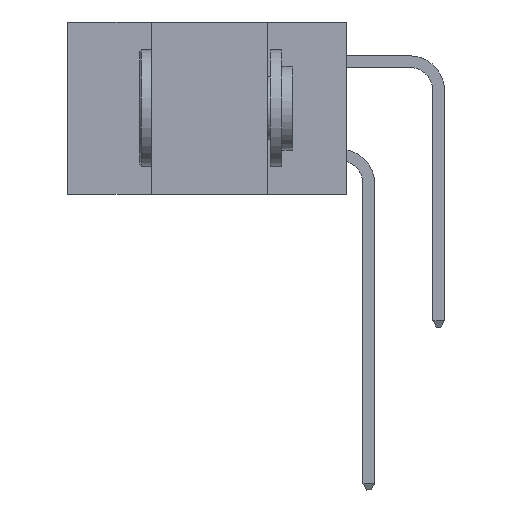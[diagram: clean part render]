
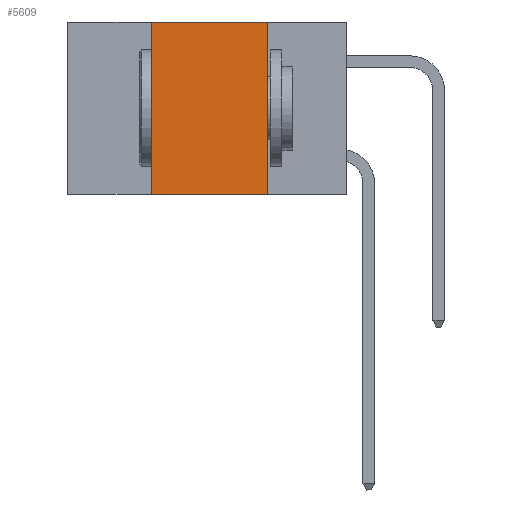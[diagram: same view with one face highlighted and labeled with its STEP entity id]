
A CAD part, left-side view. The second image highlights one B-rep face of the part: STEP entity #5609.
In plain terms, the highlighted planar face has unit normal (-1, 0, 0).
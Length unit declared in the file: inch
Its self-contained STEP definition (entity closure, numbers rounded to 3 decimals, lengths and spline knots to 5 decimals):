
#466 = EDGE_LOOP ( 'NONE', ( #12727, #6497, #14043, #6203 ) ) ;
#582 = VECTOR ( 'NONE', #4476, 39.37008 ) ;
#955 = AXIS2_PLACEMENT_3D ( 'NONE', #5650, #5880, #5606 ) ;
#1576 = CARTESIAN_POINT ( 'NONE',  ( 0., 0.17, 0. ) ) ;
#2743 = EDGE_CURVE ( 'NONE', #17007, #4978, #4250, .T. ) ;
#3438 = CARTESIAN_POINT ( 'NONE',  ( 0., 0.6, 0. ) ) ;
#4250 = LINE ( 'NONE', #3438, #582 ) ;
#4476 = DIRECTION ( 'NONE',  ( 0., -1., 0. ) ) ;
#4755 = PLANE ( 'NONE',  #955 ) ;
#4770 = EDGE_CURVE ( 'NONE', #5810, #17007, #18919, .T. ) ;
#4978 = VERTEX_POINT ( 'NONE', #1576 ) ;
#5606 = DIRECTION ( 'NONE',  ( 0., 0., -1. ) ) ;
#5609 = ADVANCED_FACE ( 'NONE', ( #12889 ), #4755, .F. ) ;
#5642 = CARTESIAN_POINT ( 'NONE',  ( 0., 0.6, -0.37 ) ) ;
#5650 = CARTESIAN_POINT ( 'NONE',  ( 0., 0.6, 0. ) ) ;
#5810 = VERTEX_POINT ( 'NONE', #12494 ) ;
#5880 = DIRECTION ( 'NONE',  ( 1., 0., 0. ) ) ;
#6203 = ORIENTED_EDGE ( 'NONE', *, *, #15522, .T. ) ;
#6497 = ORIENTED_EDGE ( 'NONE', *, *, #2743, .F. ) ;
#7171 = VECTOR ( 'NONE', #14368, 39.37008 ) ;
#7497 = VECTOR ( 'NONE', #12065, 39.37008 ) ;
#10044 = CARTESIAN_POINT ( 'NONE',  ( 0., 0.42, 0. ) ) ;
#10704 = VERTEX_POINT ( 'NONE', #15849 ) ;
#11050 = LINE ( 'NONE', #5642, #7171 ) ;
#11781 = LINE ( 'NONE', #17312, #18914 ) ;
#11841 = CARTESIAN_POINT ( 'NONE',  ( 0., 0.42, 0. ) ) ;
#12065 = DIRECTION ( 'NONE',  ( 0., 0., 1. ) ) ;
#12494 = CARTESIAN_POINT ( 'NONE',  ( 0., 0.42, -0.37 ) ) ;
#12727 = ORIENTED_EDGE ( 'NONE', *, *, #18798, .F. ) ;
#12889 = FACE_OUTER_BOUND ( 'NONE', #466, .T. ) ;
#14043 = ORIENTED_EDGE ( 'NONE', *, *, #4770, .F. ) ;
#14368 = DIRECTION ( 'NONE',  ( 0., -1., 0. ) ) ;
#15522 = EDGE_CURVE ( 'NONE', #5810, #10704, #11050, .T. ) ;
#15849 = CARTESIAN_POINT ( 'NONE',  ( 0., 0.17, -0.37 ) ) ;
#17007 = VERTEX_POINT ( 'NONE', #11841 ) ;
#17312 = CARTESIAN_POINT ( 'NONE',  ( 0., 0.17, 0. ) ) ;
#18766 = DIRECTION ( 'NONE',  ( 0., 0., -1. ) ) ;
#18798 = EDGE_CURVE ( 'NONE', #4978, #10704, #11781, .T. ) ;
#18914 = VECTOR ( 'NONE', #18766, 39.37008 ) ;
#18919 = LINE ( 'NONE', #10044, #7497 ) ;
